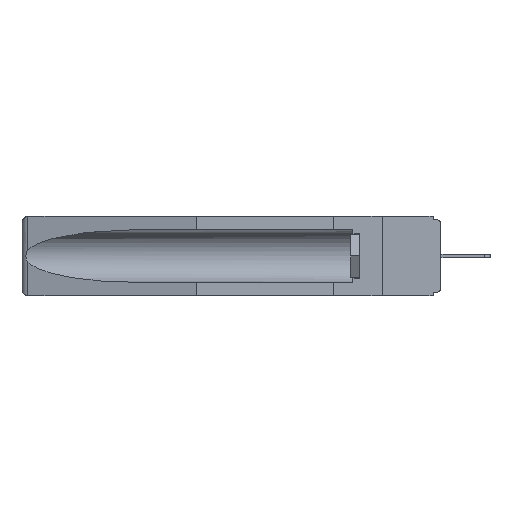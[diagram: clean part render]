
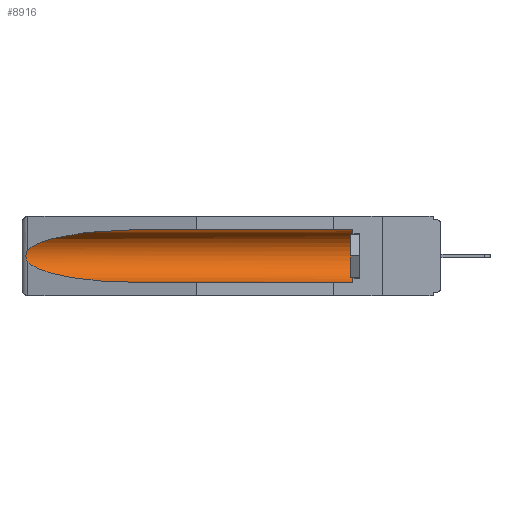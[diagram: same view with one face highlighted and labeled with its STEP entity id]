
A CAD part, left-side view. The second image highlights one B-rep face of the part: STEP entity #8916.
In plain terms, the highlighted cylindrical face has radius 2.857 mm (diameter 5.715 mm), a partial arc.
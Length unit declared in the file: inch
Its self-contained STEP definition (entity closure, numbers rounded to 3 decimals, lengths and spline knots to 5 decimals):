
#598 =( BOUNDED_CURVE ( )  B_SPLINE_CURVE ( 3, ( #2114, #8755, #12543, #4892 ),
 .UNSPECIFIED., .F., .F. ) 
 B_SPLINE_CURVE_WITH_KNOTS ( ( 4, 4 ),
 ( 4.71239, 6.08839 ),
 .UNSPECIFIED. ) 
 CURVE ( )  GEOMETRIC_REPRESENTATION_ITEM ( )  RATIONAL_B_SPLINE_CURVE ( ( 1., 0.848, 0.848, 1. ) ) 
 REPRESENTATION_ITEM ( '' )  );
#711 = CYLINDRICAL_SURFACE ( 'NONE', #16300, 0.1125 ) ;
#2055 = ORIENTED_EDGE ( 'NONE', *, *, #2638, .T. ) ;
#2089 = CARTESIAN_POINT ( 'NONE',  ( 0.26537, 1.52718, -0.14972 ) ) ;
#2114 = CARTESIAN_POINT ( 'NONE',  ( 0.155, 1.07973, -0.059 ) ) ;
#2286 = VERTEX_POINT ( 'NONE', #5595 ) ;
#2426 = AXIS2_PLACEMENT_3D ( 'NONE', #7487, #16255, #8777 ) ;
#2638 = EDGE_CURVE ( 'NONE', #8101, #8633, #10106, .T. ) ;
#2706 = LINE ( 'NONE', #3066, #5865 ) ;
#2952 = CARTESIAN_POINT ( 'NONE',  ( 0.26537, 1.52718, -0.19328 ) ) ;
#2990 = CARTESIAN_POINT ( 'NONE',  ( 0.26597, 1.5296, -0.19026 ) ) ;
#3009 = VERTEX_POINT ( 'NONE', #13506 ) ;
#3026 = CARTESIAN_POINT ( 'NONE',  ( 0.26655, 1.53094, -0.18657 ) ) ;
#3066 = CARTESIAN_POINT ( 'NONE',  ( 0.155, -0.30754, -0.059 ) ) ;
#3329 = ORIENTED_EDGE ( 'NONE', *, *, #12209, .T. ) ;
#3939 = CARTESIAN_POINT ( 'NONE',  ( 0.26537, 1.52718, -0.19328 ) ) ;
#4169 = DIRECTION ( 'NONE',  ( 0., 1., 0. ) ) ;
#4892 = CARTESIAN_POINT ( 'NONE',  ( 0.26537, 1.52718, -0.14972 ) ) ;
#4915 = CARTESIAN_POINT ( 'NONE',  ( 0.155, -0.30754, -0.284 ) ) ;
#5371 = CARTESIAN_POINT ( 'NONE',  ( 0.155, 0.126, -0.059 ) ) ;
#5595 = CARTESIAN_POINT ( 'NONE',  ( 0.155, 0.126, -0.284 ) ) ;
#5692 = CARTESIAN_POINT ( 'NONE',  ( 0.2673, 1.5327, -0.16383 ) ) ;
#5751 = DIRECTION ( 'NONE',  ( 0., 1., 0. ) ) ;
#5865 = VECTOR ( 'NONE', #5751, 39.37008 ) ;
#6013 = CARTESIAN_POINT ( 'NONE',  ( 0.26654, 1.53092, -0.15636 ) ) ;
#6062 = ORIENTED_EDGE ( 'NONE', *, *, #13250, .F. ) ;
#6166 = CARTESIAN_POINT ( 'NONE',  ( 0.26597, 1.52961, -0.15275 ) ) ;
#6442 = LINE ( 'NONE', #4915, #12760 ) ;
#6469 = ORIENTED_EDGE ( 'NONE', *, *, #14899, .T. ) ;
#7469 = ORIENTED_EDGE ( 'NONE', *, *, #8600, .T. ) ;
#7487 = CARTESIAN_POINT ( 'NONE',  ( 0.155, 0.126, -0.1715 ) ) ;
#7576 = CARTESIAN_POINT ( 'NONE',  ( 0.26537, 1.52718, -0.19328 ) ) ;
#7710 = VERTEX_POINT ( 'NONE', #5371 ) ;
#8101 = VERTEX_POINT ( 'NONE', #10247 ) ;
#8125 = CARTESIAN_POINT ( 'NONE',  ( 0.155, -0.30754, -0.1715 ) ) ;
#8600 = EDGE_CURVE ( 'NONE', #12350, #8101, #598, .T. ) ;
#8633 = VERTEX_POINT ( 'NONE', #7576 ) ;
#8755 = CARTESIAN_POINT ( 'NONE',  ( 0.21114, 1.30732, -0.059 ) ) ;
#8777 = DIRECTION ( 'NONE',  ( 0., 0., 1. ) ) ;
#8812 = EDGE_CURVE ( 'NONE', #8633, #3009, #15665, .T. ) ;
#8916 = ADVANCED_FACE ( 'NONE', ( #11563 ), #711, .F. ) ;
#9068 = ORIENTED_EDGE ( 'NONE', *, *, #8812, .T. ) ;
#9192 = CARTESIAN_POINT ( 'NONE',  ( 0.155, 1.07973, -0.284 ) ) ;
#9962 = CIRCLE ( 'NONE', #2426, 0.1125 ) ;
#10106 = B_SPLINE_CURVE_WITH_KNOTS ( 'NONE', 3,
 ( #2089, #6166, #6013, #5692, #10132, #13188, #14302, #3026, #2990, #2952 ),
 .UNSPECIFIED., .F., .F.,
 ( 4, 2, 2, 2, 4 ),
 ( 0., 0.00029, 0.00058, 0.00087, 0.00117 ),
 .UNSPECIFIED. ) ;
#10132 = CARTESIAN_POINT ( 'NONE',  ( 0.2675, 1.53308, -0.16763 ) ) ;
#10247 = CARTESIAN_POINT ( 'NONE',  ( 0.26537, 1.52718, -0.14972 ) ) ;
#11099 = CARTESIAN_POINT ( 'NONE',  ( 0.155, 1.07973, -0.059 ) ) ;
#11340 = DIRECTION ( 'NONE',  ( 0., 1., 0. ) ) ;
#11563 = FACE_OUTER_BOUND ( 'NONE', #14771, .T. ) ;
#12209 = EDGE_CURVE ( 'NONE', #7710, #12350, #2706, .T. ) ;
#12350 = VERTEX_POINT ( 'NONE', #11099 ) ;
#12543 = CARTESIAN_POINT ( 'NONE',  ( 0.25451, 1.48313, -0.09465 ) ) ;
#12760 = VECTOR ( 'NONE', #11340, 39.37008 ) ;
#12909 = CARTESIAN_POINT ( 'NONE',  ( 0.25451, 1.48313, -0.24835 ) ) ;
#13138 = DIRECTION ( 'NONE',  ( 0., 0., 1. ) ) ;
#13188 = CARTESIAN_POINT ( 'NONE',  ( 0.2675, 1.53308, -0.17534 ) ) ;
#13250 = EDGE_CURVE ( 'NONE', #2286, #3009, #6442, .T. ) ;
#13506 = CARTESIAN_POINT ( 'NONE',  ( 0.155, 1.07973, -0.284 ) ) ;
#14302 = CARTESIAN_POINT ( 'NONE',  ( 0.2673, 1.53269, -0.17917 ) ) ;
#14771 = EDGE_LOOP ( 'NONE', ( #7469, #2055, #9068, #6062, #6469, #3329 ) ) ;
#14899 = EDGE_CURVE ( 'NONE', #2286, #7710, #9962, .T. ) ;
#15665 =( BOUNDED_CURVE ( )  B_SPLINE_CURVE ( 3, ( #3939, #12909, #16642, #9192 ),
 .UNSPECIFIED., .F., .F. ) 
 B_SPLINE_CURVE_WITH_KNOTS ( ( 4, 4 ),
 ( 0.1948, 1.5708 ),
 .UNSPECIFIED. ) 
 CURVE ( )  GEOMETRIC_REPRESENTATION_ITEM ( )  RATIONAL_B_SPLINE_CURVE ( ( 1., 0.848, 0.848, 1. ) ) 
 REPRESENTATION_ITEM ( '' )  );
#16255 = DIRECTION ( 'NONE',  ( 0., -1., 0. ) ) ;
#16300 = AXIS2_PLACEMENT_3D ( 'NONE', #8125, #4169, #13138 ) ;
#16642 = CARTESIAN_POINT ( 'NONE',  ( 0.21114, 1.30732, -0.284 ) ) ;
